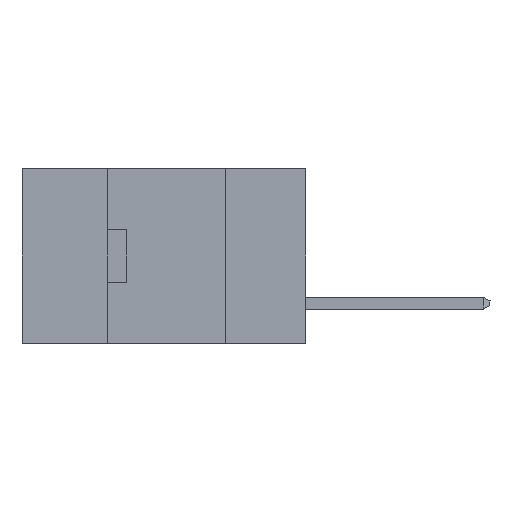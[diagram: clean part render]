
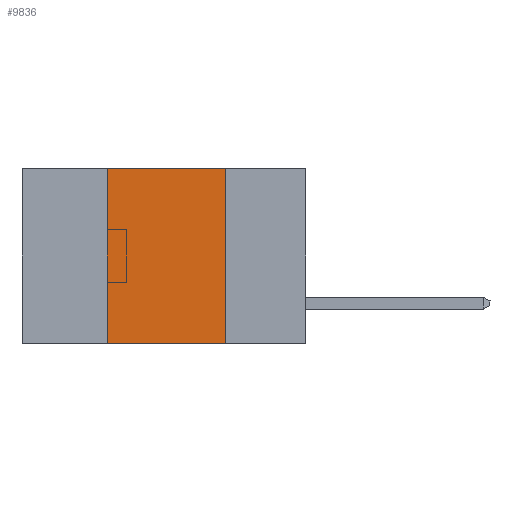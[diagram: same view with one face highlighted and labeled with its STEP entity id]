
A CAD part, left-side view. The second image highlights one B-rep face of the part: STEP entity #9836.
In plain terms, the highlighted planar face has unit normal (-1, 0, 0).
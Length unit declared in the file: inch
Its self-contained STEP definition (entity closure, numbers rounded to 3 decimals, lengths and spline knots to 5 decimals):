
#1050 = VECTOR ( 'NONE', #11836, 39.37008 ) ;
#1281 = VECTOR ( 'NONE', #20225, 39.37008 ) ;
#1783 = EDGE_LOOP ( 'NONE', ( #26482, #5099, #12536, #3469 ) ) ;
#2480 = AXIS2_PLACEMENT_3D ( 'NONE', #14657, #18967, #8754 ) ;
#2901 = EDGE_CURVE ( 'NONE', #24393, #5311, #4292, .T. ) ;
#3469 = ORIENTED_EDGE ( 'NONE', *, *, #22445, .T. ) ;
#4292 = LINE ( 'NONE', #10870, #24669 ) ;
#5099 = ORIENTED_EDGE ( 'NONE', *, *, #19590, .F. ) ;
#5311 = VERTEX_POINT ( 'NONE', #5587 ) ;
#5574 = CARTESIAN_POINT ( 'NONE',  ( 0., 0.6, -0.37 ) ) ;
#5587 = CARTESIAN_POINT ( 'NONE',  ( 0., 0.42, 0. ) ) ;
#8754 = DIRECTION ( 'NONE',  ( 0., 0., -1. ) ) ;
#9752 = LINE ( 'NONE', #22231, #1281 ) ;
#9836 = ADVANCED_FACE ( 'NONE', ( #15185 ), #12640, .F. ) ;
#10870 = CARTESIAN_POINT ( 'NONE',  ( 0., 0.42, -0.37 ) ) ;
#11617 = EDGE_CURVE ( 'NONE', #14269, #22424, #9752, .T. ) ;
#11836 = DIRECTION ( 'NONE',  ( 0., -1., 0. ) ) ;
#12273 = LINE ( 'NONE', #5574, #23911 ) ;
#12536 = ORIENTED_EDGE ( 'NONE', *, *, #2901, .F. ) ;
#12640 = PLANE ( 'NONE',  #2480 ) ;
#14023 = CARTESIAN_POINT ( 'NONE',  ( 0., 0.17, -0.37 ) ) ;
#14269 = VERTEX_POINT ( 'NONE', #26164 ) ;
#14657 = CARTESIAN_POINT ( 'NONE',  ( 0., 0.6, 0. ) ) ;
#15185 = FACE_OUTER_BOUND ( 'NONE', #1783, .T. ) ;
#18967 = DIRECTION ( 'NONE',  ( 1., 0., 0. ) ) ;
#19086 = DIRECTION ( 'NONE',  ( 0., 0., 1. ) ) ;
#19590 = EDGE_CURVE ( 'NONE', #5311, #14269, #21394, .T. ) ;
#19907 = CARTESIAN_POINT ( 'NONE',  ( 0., 0.6, 0. ) ) ;
#20225 = DIRECTION ( 'NONE',  ( 0., 0., -1. ) ) ;
#20619 = CARTESIAN_POINT ( 'NONE',  ( 0., 0.42, -0.37 ) ) ;
#21394 = LINE ( 'NONE', #19907, #1050 ) ;
#21957 = DIRECTION ( 'NONE',  ( 0., -1., 0. ) ) ;
#22231 = CARTESIAN_POINT ( 'NONE',  ( 0., 0.17, -0.37 ) ) ;
#22424 = VERTEX_POINT ( 'NONE', #14023 ) ;
#22445 = EDGE_CURVE ( 'NONE', #24393, #22424, #12273, .T. ) ;
#23911 = VECTOR ( 'NONE', #21957, 39.37008 ) ;
#24393 = VERTEX_POINT ( 'NONE', #20619 ) ;
#24669 = VECTOR ( 'NONE', #19086, 39.37008 ) ;
#26164 = CARTESIAN_POINT ( 'NONE',  ( 0., 0.17, 0. ) ) ;
#26482 = ORIENTED_EDGE ( 'NONE', *, *, #11617, .F. ) ;
